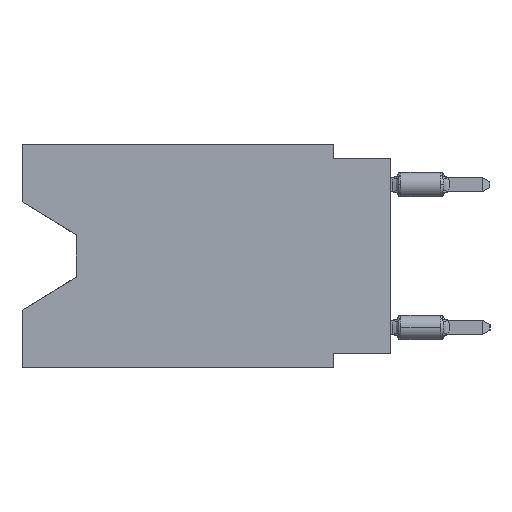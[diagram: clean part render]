
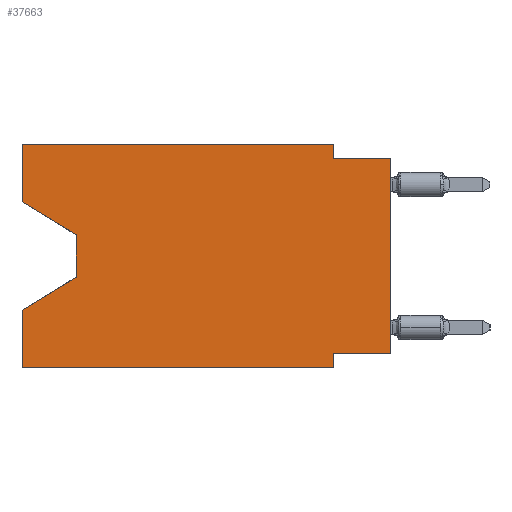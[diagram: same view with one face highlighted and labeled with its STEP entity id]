
A CAD part, left-side view. The second image highlights one B-rep face of the part: STEP entity #37663.
In plain terms, the highlighted planar face has unit normal (-1, 0, 0).
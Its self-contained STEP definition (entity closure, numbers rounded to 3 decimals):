
#912 = VECTOR ( 'NONE', #37215, 1000. ) ;
#1618 = DIRECTION ( 'NONE',  ( 0., 0., -1. ) ) ;
#1712 = LINE ( 'NONE', #25256, #16925 ) ;
#1802 = VERTEX_POINT ( 'NONE', #3129 ) ;
#2179 = LINE ( 'NONE', #31363, #14987 ) ;
#2254 = AXIS2_PLACEMENT_3D ( 'NONE', #7185, #31152, #6804 ) ;
#2506 = VECTOR ( 'NONE', #29522, 1000. ) ;
#3129 = CARTESIAN_POINT ( 'NONE',  ( 0., 16.383, -9.906 ) ) ;
#3530 = EDGE_CURVE ( 'NONE', #1802, #31086, #8838, .T. ) ;
#3937 = VERTEX_POINT ( 'NONE', #35762 ) ;
#3961 = VECTOR ( 'NONE', #37601, 1000. ) ;
#4169 = ORIENTED_EDGE ( 'NONE', *, *, #26516, .F. ) ;
#4179 = ORIENTED_EDGE ( 'NONE', *, *, #37859, .T. ) ;
#5782 = VECTOR ( 'NONE', #11943, 1000. ) ;
#5977 = LINE ( 'NONE', #9412, #2506 ) ;
#6186 = VECTOR ( 'NONE', #1618, 1000. ) ;
#6804 = DIRECTION ( 'NONE',  ( 0., 0., -1. ) ) ;
#7185 = CARTESIAN_POINT ( 'NONE',  ( 0., 16.383, 0. ) ) ;
#7531 = VERTEX_POINT ( 'NONE', #9669 ) ;
#7594 = VERTEX_POINT ( 'NONE', #21263 ) ;
#7867 = VERTEX_POINT ( 'NONE', #22986 ) ;
#7869 = ORIENTED_EDGE ( 'NONE', *, *, #28606, .T. ) ;
#8838 = LINE ( 'NONE', #20049, #19902 ) ;
#9241 = CARTESIAN_POINT ( 'NONE',  ( 0., 16.383, 0. ) ) ;
#9412 = CARTESIAN_POINT ( 'NONE',  ( 0., 0., -9.271 ) ) ;
#9669 = CARTESIAN_POINT ( 'NONE',  ( 0., 2.54, 0. ) ) ;
#10457 = VECTOR ( 'NONE', #32127, 1000. ) ;
#10473 = VERTEX_POINT ( 'NONE', #22697 ) ;
#10716 = DIRECTION ( 'NONE',  ( 0., -1., 0. ) ) ;
#11943 = DIRECTION ( 'NONE',  ( 0., 0., 1. ) ) ;
#12323 = EDGE_CURVE ( 'NONE', #29119, #7867, #27252, .T. ) ;
#12804 = ORIENTED_EDGE ( 'NONE', *, *, #36881, .T. ) ;
#13804 = CARTESIAN_POINT ( 'NONE',  ( 0., 0., -9.271 ) ) ;
#14987 = VECTOR ( 'NONE', #22640, 1000. ) ;
#15351 = CARTESIAN_POINT ( 'NONE',  ( 0., 2.54, -9.906 ) ) ;
#15612 = ORIENTED_EDGE ( 'NONE', *, *, #27891, .F. ) ;
#16163 = ORIENTED_EDGE ( 'NONE', *, *, #12323, .T. ) ;
#16434 = VECTOR ( 'NONE', #29567, 1000. ) ;
#16925 = VECTOR ( 'NONE', #24880, 1000. ) ;
#17419 = CARTESIAN_POINT ( 'NONE',  ( 0., 13.97, -4.013 ) ) ;
#17775 = CARTESIAN_POINT ( 'NONE',  ( 0., 16.383, -2.546 ) ) ;
#18861 = VECTOR ( 'NONE', #31074, 1000. ) ;
#19902 = VECTOR ( 'NONE', #28755, 1000. ) ;
#20049 = CARTESIAN_POINT ( 'NONE',  ( 0., 16.383, -9.906 ) ) ;
#20317 = CARTESIAN_POINT ( 'NONE',  ( 0., 0., -0.635 ) ) ;
#20401 = CARTESIAN_POINT ( 'NONE',  ( 0., 16.383, -2.546 ) ) ;
#21263 = CARTESIAN_POINT ( 'NONE',  ( 0., 16.383, 0. ) ) ;
#21485 = PLANE ( 'NONE',  #2254 ) ;
#22158 = CARTESIAN_POINT ( 'NONE',  ( 0., 0., 0. ) ) ;
#22433 = VECTOR ( 'NONE', #10716, 1000. ) ;
#22640 = DIRECTION ( 'NONE',  ( 0., 0., -1. ) ) ;
#22697 = CARTESIAN_POINT ( 'NONE',  ( 0., 2.54, -0.635 ) ) ;
#22969 = ORIENTED_EDGE ( 'NONE', *, *, #37123, .F. ) ;
#22986 = CARTESIAN_POINT ( 'NONE',  ( 0., 0., -0.635 ) ) ;
#23271 = CARTESIAN_POINT ( 'NONE',  ( 0., 2.54, 0. ) ) ;
#23479 = CARTESIAN_POINT ( 'NONE',  ( 0., 13.97, -5.893 ) ) ;
#24880 = DIRECTION ( 'NONE',  ( 0., 0.855, -0.519 ) ) ;
#25212 = LINE ( 'NONE', #37211, #22433 ) ;
#25256 = CARTESIAN_POINT ( 'NONE',  ( 0., 13.97, -5.893 ) ) ;
#25400 = CARTESIAN_POINT ( 'NONE',  ( 0., 16.383, 0. ) ) ;
#25690 = CARTESIAN_POINT ( 'NONE',  ( 0., 16.383, -7.36 ) ) ;
#26516 = EDGE_CURVE ( 'NONE', #3937, #31086, #2179, .T. ) ;
#26974 = VERTEX_POINT ( 'NONE', #25690 ) ;
#27215 = EDGE_CURVE ( 'NONE', #36208, #7594, #27604, .T. ) ;
#27252 = LINE ( 'NONE', #22158, #18861 ) ;
#27604 = LINE ( 'NONE', #9241, #5782 ) ;
#27698 = EDGE_CURVE ( 'NONE', #7594, #7531, #25212, .T. ) ;
#27891 = EDGE_CURVE ( 'NONE', #7531, #10473, #34311, .T. ) ;
#27934 = ORIENTED_EDGE ( 'NONE', *, *, #33457, .F. ) ;
#28079 = LINE ( 'NONE', #33890, #6186 ) ;
#28270 = ORIENTED_EDGE ( 'NONE', *, *, #29088, .F. ) ;
#28313 = LINE ( 'NONE', #25400, #912 ) ;
#28590 = EDGE_LOOP ( 'NONE', ( #4179, #12804, #7869, #28270, #30379, #4169, #27934, #16163, #22969, #15612, #32923, #35831 ) ) ;
#28606 = EDGE_CURVE ( 'NONE', #30925, #26974, #1712, .T. ) ;
#28755 = DIRECTION ( 'NONE',  ( 0., -1., 0. ) ) ;
#29088 = EDGE_CURVE ( 'NONE', #1802, #26974, #28313, .T. ) ;
#29119 = VERTEX_POINT ( 'NONE', #13804 ) ;
#29522 = DIRECTION ( 'NONE',  ( 0., 1., 0. ) ) ;
#29567 = DIRECTION ( 'NONE',  ( 0., -0.855, -0.519 ) ) ;
#30379 = ORIENTED_EDGE ( 'NONE', *, *, #3530, .T. ) ;
#30925 = VERTEX_POINT ( 'NONE', #23479 ) ;
#31074 = DIRECTION ( 'NONE',  ( 0., 0., 1. ) ) ;
#31086 = VERTEX_POINT ( 'NONE', #15351 ) ;
#31152 = DIRECTION ( 'NONE',  ( 1., 0., 0. ) ) ;
#31363 = CARTESIAN_POINT ( 'NONE',  ( 0., 2.54, -9.906 ) ) ;
#32127 = DIRECTION ( 'NONE',  ( 0., -1., 0. ) ) ;
#32492 = LINE ( 'NONE', #17775, #16434 ) ;
#32923 = ORIENTED_EDGE ( 'NONE', *, *, #27698, .F. ) ;
#33457 = EDGE_CURVE ( 'NONE', #29119, #3937, #5977, .T. ) ;
#33668 = FACE_OUTER_BOUND ( 'NONE', #28590, .T. ) ;
#33890 = CARTESIAN_POINT ( 'NONE',  ( 0., 13.97, -4.013 ) ) ;
#34311 = LINE ( 'NONE', #23271, #3961 ) ;
#35031 = LINE ( 'NONE', #20317, #10457 ) ;
#35762 = CARTESIAN_POINT ( 'NONE',  ( 0., 2.54, -9.271 ) ) ;
#35831 = ORIENTED_EDGE ( 'NONE', *, *, #27215, .F. ) ;
#36208 = VERTEX_POINT ( 'NONE', #20401 ) ;
#36881 = EDGE_CURVE ( 'NONE', #37028, #30925, #28079, .T. ) ;
#37028 = VERTEX_POINT ( 'NONE', #17419 ) ;
#37123 = EDGE_CURVE ( 'NONE', #10473, #7867, #35031, .T. ) ;
#37211 = CARTESIAN_POINT ( 'NONE',  ( 0., 16.383, 0. ) ) ;
#37215 = DIRECTION ( 'NONE',  ( 0., 0., 1. ) ) ;
#37601 = DIRECTION ( 'NONE',  ( 0., 0., -1. ) ) ;
#37663 = ADVANCED_FACE ( 'NONE', ( #33668 ), #21485, .F. ) ;
#37859 = EDGE_CURVE ( 'NONE', #36208, #37028, #32492, .T. ) ;
